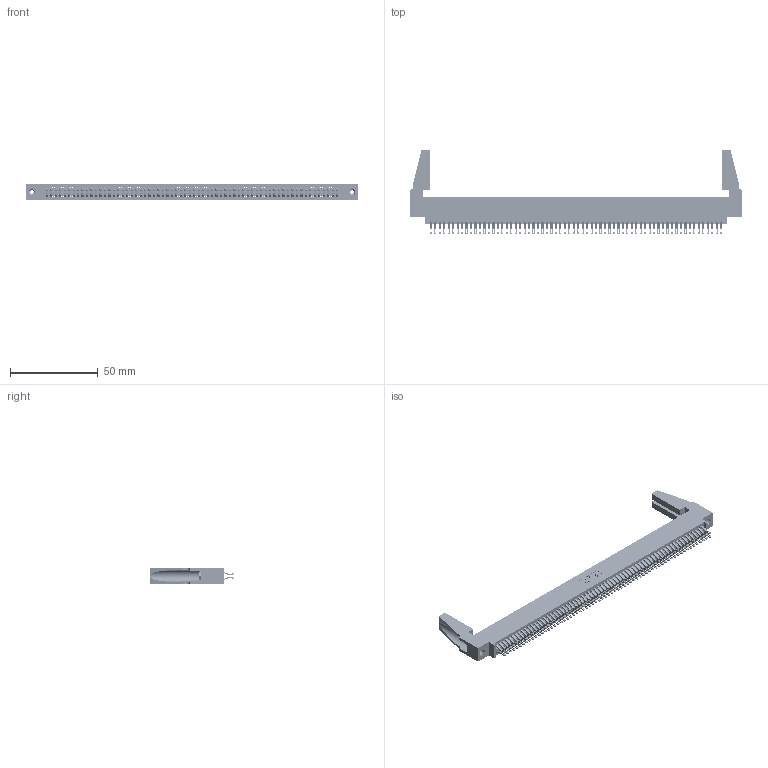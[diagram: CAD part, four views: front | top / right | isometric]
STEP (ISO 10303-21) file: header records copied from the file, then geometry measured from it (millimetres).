
FILE_DESCRIPTION (( 'STEP AP203' ), '1' );
FILE_NAME ('345-132-555-888.STEP', '2019-11-07T22:24:26', ( '' ), ( '' ), 'SwSTEP 2.0', 'SolidWorks 2016', '' );
FILE_SCHEMA (( 'CONFIG_CONTROL_DESIGN' ));
Length unit declared in the file: inch
Products named in the file (5): 345-132-555-888; 345-250-001_345-250-001-102; 345-292-001_555 Tail; 345 Part_0.170 Offset - 0.156 Dia-TH; 345-220-078_345-220-088
Assembly tree (137 placements, depth 2):
  345-132-555-888
    345 Part_0.170 Offset - 0.156 Dia-TH
    345-292-001_555 Tail  x132
    345-250-001_345-250-001-102  x2
    345-220-078_345-220-088  x2
Bounding box: 188.87 x 48.31 x 9.4 mm (x, y, z)
Volume: 22092.2 mm3; surface area: 32910.4 mm2
Topology: 137 solids, 137 shells, 7646 faces, 24031 edges, 16010 vertices
Faces by surface type: plane 4248, cylinder 3382, cone 12, torus 4
Entity records: 51160 total; most frequent: CARTESIAN_POINT 8584, ORIENTED_EDGE 8448, DIRECTION 7512, EDGE_CURVE 4224, VECTOR 3766, LINE 3766, VERTEX_POINT 2810, AXIS2_PLACEMENT_3D 1873
